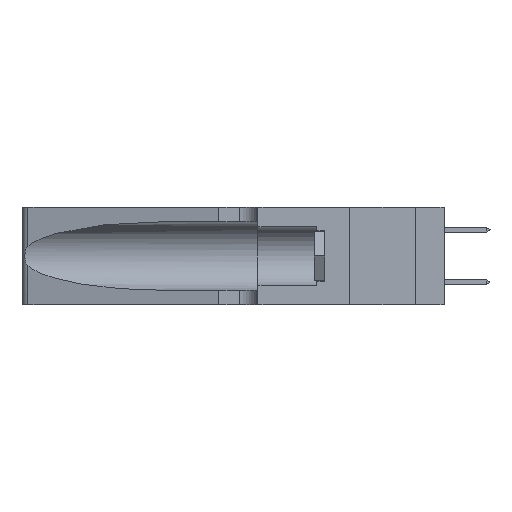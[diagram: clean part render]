
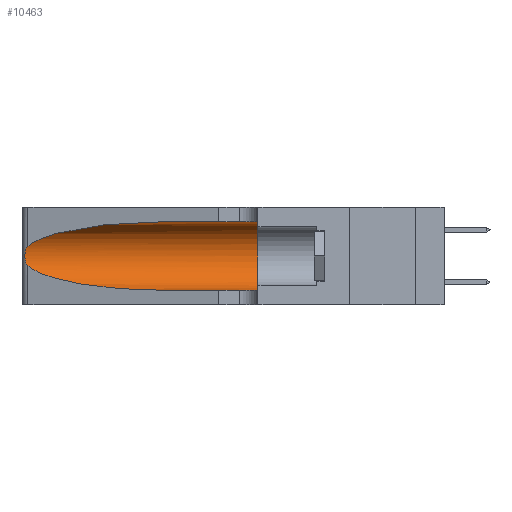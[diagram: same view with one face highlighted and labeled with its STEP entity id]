
A CAD part, left-side view. The second image highlights one B-rep face of the part: STEP entity #10463.
In plain terms, the highlighted cylindrical face has radius 3.308 mm (diameter 6.617 mm), a partial arc.
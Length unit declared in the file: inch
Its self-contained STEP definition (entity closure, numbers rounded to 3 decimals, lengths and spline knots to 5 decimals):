
#2030 =( BOUNDED_CURVE ( )  B_SPLINE_CURVE ( 3, ( #38771, #6106, #12468, #36362 ),
 .UNSPECIFIED., .F., .T. ) 
 B_SPLINE_CURVE_WITH_KNOTS ( ( 4, 4 ),
 ( 3.44316, 4.71239 ),
 .UNSPECIFIED. ) 
 CURVE ( )  GEOMETRIC_REPRESENTATION_ITEM ( )  RATIONAL_B_SPLINE_CURVE ( ( 1., 0.87, 0.87, 1. ) ) 
 REPRESENTATION_ITEM ( '' )  );
#3695 = CARTESIAN_POINT ( 'NONE',  ( 0.1305, 0.72297, 0.31525 ) ) ;
#3713 = VERTEX_POINT ( 'NONE', #28318 ) ;
#4282 = VECTOR ( 'NONE', #37488, 39.37008 ) ;
#4938 = FACE_OUTER_BOUND ( 'NONE', #14245, .T. ) ;
#5555 = ORIENTED_EDGE ( 'NONE', *, *, #10541, .F. ) ;
#5764 = CARTESIAN_POINT ( 'NONE',  ( 0.25487, 1.22718, 0.22369 ) ) ;
#6106 = CARTESIAN_POINT ( 'NONE',  ( 0.2373, 1.15595, 0.08982 ) ) ;
#6130 = AXIS2_PLACEMENT_3D ( 'NONE', #32719, #26727, #33102 ) ;
#6691 = DIRECTION ( 'NONE',  ( 0., 0., 1. ) ) ;
#6826 = CARTESIAN_POINT ( 'NONE',  ( 0.1305, 0.35, 0.185 ) ) ;
#8274 = CARTESIAN_POINT ( 'NONE',  ( 0.25639, 1.23184, 0.21858 ) ) ;
#8714 = AXIS2_PLACEMENT_3D ( 'NONE', #6826, #15954, #6691 ) ;
#9564 = VERTEX_POINT ( 'NONE', #25327 ) ;
#10463 = ADVANCED_FACE ( 'NONE', ( #4938 ), #30552, .F. ) ;
#10541 = EDGE_CURVE ( 'NONE', #26344, #3713, #32441, .T. ) ;
#11486 = VERTEX_POINT ( 'NONE', #25806 ) ;
#11624 = DIRECTION ( 'NONE',  ( 0., -1., 0. ) ) ;
#11712 = ORIENTED_EDGE ( 'NONE', *, *, #38877, .T. ) ;
#12138 = VERTEX_POINT ( 'NONE', #16459 ) ;
#12468 = CARTESIAN_POINT ( 'NONE',  ( 0.18966, 0.96281, 0.05475 ) ) ;
#12554 = VERTEX_POINT ( 'NONE', #30927 ) ;
#14245 = EDGE_LOOP ( 'NONE', ( #15819, #11712, #39112, #36876, #33854, #5555 ) ) ;
#14624 = CARTESIAN_POINT ( 'NONE',  ( 0.25787, 1.23484, 0.2124 ) ) ;
#14782 = CIRCLE ( 'NONE', #8714, 0.13025 ) ;
#14886 = CARTESIAN_POINT ( 'NONE',  ( 0.25854, 1.2359, 0.20912 ) ) ;
#15819 = ORIENTED_EDGE ( 'NONE', *, *, #25334, .T. ) ;
#15954 = DIRECTION ( 'NONE',  ( 0., 1., 0. ) ) ;
#16358 =( BOUNDED_CURVE ( )  B_SPLINE_CURVE ( 3, ( #35063, #29094, #32271, #28843 ),
 .UNSPECIFIED., .F., .F. ) 
 B_SPLINE_CURVE_WITH_KNOTS ( ( 4, 4 ),
 ( 1.5708, 2.84003 ),
 .UNSPECIFIED. ) 
 CURVE ( )  GEOMETRIC_REPRESENTATION_ITEM ( )  RATIONAL_B_SPLINE_CURVE ( ( 1., 0.87, 0.87, 1. ) ) 
 REPRESENTATION_ITEM ( '' )  );
#16459 = CARTESIAN_POINT ( 'NONE',  ( 0.1305, 0.72297, 0.05475 ) ) ;
#17532 = CARTESIAN_POINT ( 'NONE',  ( 0.25639, 1.23186, 0.15144 ) ) ;
#20325 = CARTESIAN_POINT ( 'NONE',  ( 0.26075, 1.23896, 0.178 ) ) ;
#20587 = CARTESIAN_POINT ( 'NONE',  ( 0.25555, 1.22993, 0.14849 ) ) ;
#22669 = B_SPLINE_CURVE_WITH_KNOTS ( 'NONE', 3,
 ( #5764, #26960, #8274, #14624, #14886, #23531, #36002, #20325, #29785, #26575, #32692, #17532, #20587, #26699 ),
 .UNSPECIFIED., .F., .F.,
 ( 4, 2, 2, 2, 2, 2, 4 ),
 ( 0., 0.00027, 0.00053, 0.00107, 0.0016, 0.00187, 0.00214 ),
 .UNSPECIFIED. ) ;
#23531 = CARTESIAN_POINT ( 'NONE',  ( 0.26018, 1.23835, 0.19895 ) ) ;
#25003 = CARTESIAN_POINT ( 'NONE',  ( 0.1305, 1.61858, 0.05475 ) ) ;
#25327 = CARTESIAN_POINT ( 'NONE',  ( 0.1305, 0.35, 0.05475 ) ) ;
#25334 = EDGE_CURVE ( 'NONE', #26344, #12554, #16358, .T. ) ;
#25806 = CARTESIAN_POINT ( 'NONE',  ( 0.25487, 1.22718, 0.14631 ) ) ;
#26344 = VERTEX_POINT ( 'NONE', #3695 ) ;
#26575 = CARTESIAN_POINT ( 'NONE',  ( 0.25856, 1.23593, 0.16098 ) ) ;
#26699 = CARTESIAN_POINT ( 'NONE',  ( 0.25487, 1.22718, 0.14631 ) ) ;
#26727 = DIRECTION ( 'NONE',  ( 0., -1., 0. ) ) ;
#26960 = CARTESIAN_POINT ( 'NONE',  ( 0.25555, 1.22994, 0.2215 ) ) ;
#28318 = CARTESIAN_POINT ( 'NONE',  ( 0.1305, 0.35, 0.31525 ) ) ;
#28654 = VECTOR ( 'NONE', #11624, 39.37008 ) ;
#28843 = CARTESIAN_POINT ( 'NONE',  ( 0.25487, 1.22718, 0.22369 ) ) ;
#29094 = CARTESIAN_POINT ( 'NONE',  ( 0.18966, 0.96281, 0.31525 ) ) ;
#29285 = EDGE_CURVE ( 'NONE', #12138, #9564, #36104, .T. ) ;
#29785 = CARTESIAN_POINT ( 'NONE',  ( 0.26017, 1.23833, 0.17102 ) ) ;
#29815 = CARTESIAN_POINT ( 'NONE',  ( 0.1305, 1.61858, 0.31525 ) ) ;
#30552 = CYLINDRICAL_SURFACE ( 'NONE', #6130, 0.13025 ) ;
#30927 = CARTESIAN_POINT ( 'NONE',  ( 0.25487, 1.22718, 0.22369 ) ) ;
#32271 = CARTESIAN_POINT ( 'NONE',  ( 0.2373, 1.15595, 0.28018 ) ) ;
#32441 = LINE ( 'NONE', #29815, #28654 ) ;
#32692 = CARTESIAN_POINT ( 'NONE',  ( 0.25789, 1.23486, 0.15765 ) ) ;
#32719 = CARTESIAN_POINT ( 'NONE',  ( 0.1305, 1.61858, 0.185 ) ) ;
#33102 = DIRECTION ( 'NONE',  ( 0., 0., -1. ) ) ;
#33854 = ORIENTED_EDGE ( 'NONE', *, *, #35193, .F. ) ;
#34624 = EDGE_CURVE ( 'NONE', #11486, #12138, #2030, .T. ) ;
#35063 = CARTESIAN_POINT ( 'NONE',  ( 0.1305, 0.72297, 0.31525 ) ) ;
#35193 = EDGE_CURVE ( 'NONE', #3713, #9564, #14782, .T. ) ;
#36002 = CARTESIAN_POINT ( 'NONE',  ( 0.26075, 1.23896, 0.19203 ) ) ;
#36104 = LINE ( 'NONE', #25003, #4282 ) ;
#36362 = CARTESIAN_POINT ( 'NONE',  ( 0.1305, 0.72297, 0.05475 ) ) ;
#36876 = ORIENTED_EDGE ( 'NONE', *, *, #29285, .T. ) ;
#37488 = DIRECTION ( 'NONE',  ( 0., -1., 0. ) ) ;
#38771 = CARTESIAN_POINT ( 'NONE',  ( 0.25487, 1.22718, 0.14631 ) ) ;
#38877 = EDGE_CURVE ( 'NONE', #12554, #11486, #22669, .T. ) ;
#39112 = ORIENTED_EDGE ( 'NONE', *, *, #34624, .T. ) ;
